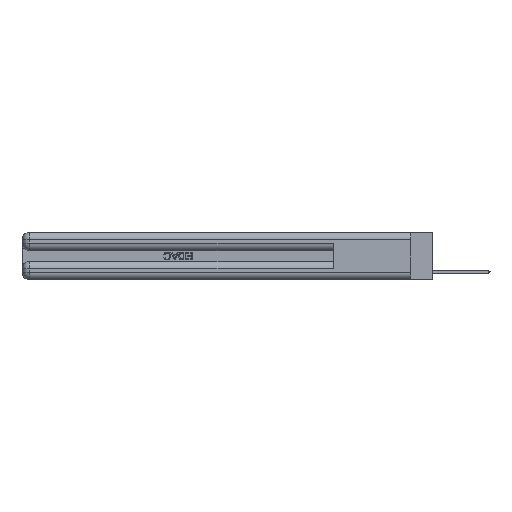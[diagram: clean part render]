
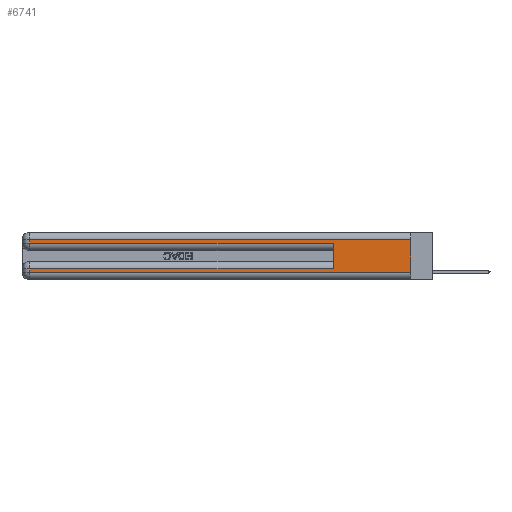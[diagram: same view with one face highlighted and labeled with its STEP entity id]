
A CAD part, left-side view. The second image highlights one B-rep face of the part: STEP entity #6741.
In plain terms, the highlighted planar face has unit normal (-1, 0, 0).
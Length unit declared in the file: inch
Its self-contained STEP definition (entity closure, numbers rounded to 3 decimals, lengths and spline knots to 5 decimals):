
#21 = CARTESIAN_POINT ( 'NONE',  ( 0., 2.94, 0.06 ) ) ;
#258 = LINE ( 'NONE', #3412, #27364 ) ;
#299 = CARTESIAN_POINT ( 'NONE',  ( 0., 0., 0.37 ) ) ;
#485 = CARTESIAN_POINT ( 'NONE',  ( 0., 0., 0.285 ) ) ;
#514 = CARTESIAN_POINT ( 'NONE',  ( 0., 0.6, 0.085 ) ) ;
#777 = DIRECTION ( 'NONE',  ( 0., -1., 0. ) ) ;
#1890 = AXIS2_PLACEMENT_3D ( 'NONE', #299, #24243, #34608 ) ;
#2693 = ORIENTED_EDGE ( 'NONE', *, *, #22462, .T. ) ;
#2773 = PLANE ( 'NONE',  #1890 ) ;
#3412 = CARTESIAN_POINT ( 'NONE',  ( 0., 0., 0.06 ) ) ;
#4109 = ORIENTED_EDGE ( 'NONE', *, *, #8827, .T. ) ;
#4467 = EDGE_CURVE ( 'NONE', #25784, #27739, #9883, .T. ) ;
#4496 = EDGE_CURVE ( 'NONE', #27739, #13645, #23273, .T. ) ;
#4881 = ORIENTED_EDGE ( 'NONE', *, *, #27232, .T. ) ;
#4959 = CARTESIAN_POINT ( 'NONE',  ( 0., 0.6, 0.145 ) ) ;
#6175 = VERTEX_POINT ( 'NONE', #33785 ) ;
#6741 = ADVANCED_FACE ( 'NONE', ( #26877 ), #2773, .F. ) ;
#7100 = VERTEX_POINT ( 'NONE', #25792 ) ;
#7932 = LINE ( 'NONE', #18882, #21237 ) ;
#8827 = EDGE_CURVE ( 'NONE', #24576, #6175, #12363, .T. ) ;
#8873 = CARTESIAN_POINT ( 'NONE',  ( 0., 2.94, 0.285 ) ) ;
#8901 = CARTESIAN_POINT ( 'NONE',  ( 0., 0., 0.31 ) ) ;
#9057 = EDGE_CURVE ( 'NONE', #25784, #22055, #12885, .T. ) ;
#9883 = LINE ( 'NONE', #25912, #31658 ) ;
#10582 = DIRECTION ( 'NONE',  ( 0., 0., 1. ) ) ;
#10907 = CARTESIAN_POINT ( 'NONE',  ( 0., 0.6, 0.285 ) ) ;
#11435 = VECTOR ( 'NONE', #34506, 39.37008 ) ;
#12363 = LINE ( 'NONE', #8901, #18682 ) ;
#12503 = VECTOR ( 'NONE', #10582, 39.37008 ) ;
#12885 = LINE ( 'NONE', #4959, #12503 ) ;
#13645 = VERTEX_POINT ( 'NONE', #21 ) ;
#14073 = CARTESIAN_POINT ( 'NONE',  ( 0., 2.94, 0.085 ) ) ;
#14557 = EDGE_CURVE ( 'NONE', #24576, #7100, #31908, .T. ) ;
#15036 = EDGE_CURVE ( 'NONE', #6175, #28555, #7932, .T. ) ;
#15738 = CARTESIAN_POINT ( 'NONE',  ( 0., 0., 0.37 ) ) ;
#18682 = VECTOR ( 'NONE', #19846, 39.37008 ) ;
#18882 = CARTESIAN_POINT ( 'NONE',  ( 0., 2.94, 0.37 ) ) ;
#19846 = DIRECTION ( 'NONE',  ( 0., 1., 0. ) ) ;
#20652 = VECTOR ( 'NONE', #29452, 39.37008 ) ;
#21237 = VECTOR ( 'NONE', #29409, 39.37008 ) ;
#21818 = CARTESIAN_POINT ( 'NONE',  ( 0., 0., 0.31 ) ) ;
#22055 = VERTEX_POINT ( 'NONE', #10907 ) ;
#22462 = EDGE_CURVE ( 'NONE', #28555, #22055, #24768, .T. ) ;
#22673 = ORIENTED_EDGE ( 'NONE', *, *, #14557, .F. ) ;
#23273 = LINE ( 'NONE', #23795, #11435 ) ;
#23435 = DIRECTION ( 'NONE',  ( 0., 1., 0. ) ) ;
#23795 = CARTESIAN_POINT ( 'NONE',  ( 0., 2.94, 0.37 ) ) ;
#24243 = DIRECTION ( 'NONE',  ( 1., 0., 0. ) ) ;
#24297 = VECTOR ( 'NONE', #32841, 39.37008 ) ;
#24393 = ORIENTED_EDGE ( 'NONE', *, *, #4467, .T. ) ;
#24576 = VERTEX_POINT ( 'NONE', #21818 ) ;
#24768 = LINE ( 'NONE', #485, #24297 ) ;
#25784 = VERTEX_POINT ( 'NONE', #514 ) ;
#25792 = CARTESIAN_POINT ( 'NONE',  ( 0., 0., 0.06 ) ) ;
#25912 = CARTESIAN_POINT ( 'NONE',  ( 0., 0., 0.085 ) ) ;
#26877 = FACE_OUTER_BOUND ( 'NONE', #27292, .T. ) ;
#26991 = ORIENTED_EDGE ( 'NONE', *, *, #4496, .T. ) ;
#27232 = EDGE_CURVE ( 'NONE', #13645, #7100, #258, .T. ) ;
#27292 = EDGE_LOOP ( 'NONE', ( #22673, #4109, #33784, #2693, #29116, #24393, #26991, #4881 ) ) ;
#27364 = VECTOR ( 'NONE', #777, 39.37008 ) ;
#27739 = VERTEX_POINT ( 'NONE', #14073 ) ;
#28555 = VERTEX_POINT ( 'NONE', #8873 ) ;
#29116 = ORIENTED_EDGE ( 'NONE', *, *, #9057, .F. ) ;
#29409 = DIRECTION ( 'NONE',  ( 0., 0., -1. ) ) ;
#29452 = DIRECTION ( 'NONE',  ( 0., 0., -1. ) ) ;
#31658 = VECTOR ( 'NONE', #23435, 39.37008 ) ;
#31908 = LINE ( 'NONE', #15738, #20652 ) ;
#32841 = DIRECTION ( 'NONE',  ( 0., -1., 0. ) ) ;
#33784 = ORIENTED_EDGE ( 'NONE', *, *, #15036, .T. ) ;
#33785 = CARTESIAN_POINT ( 'NONE',  ( 0., 2.94, 0.31 ) ) ;
#34506 = DIRECTION ( 'NONE',  ( 0., 0., -1. ) ) ;
#34608 = DIRECTION ( 'NONE',  ( 0., 0., -1. ) ) ;
